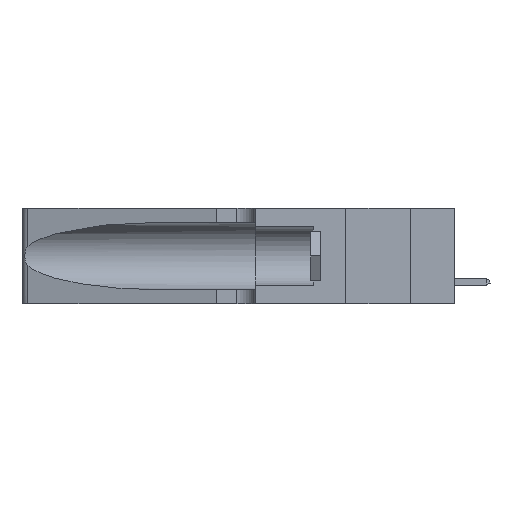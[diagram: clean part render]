
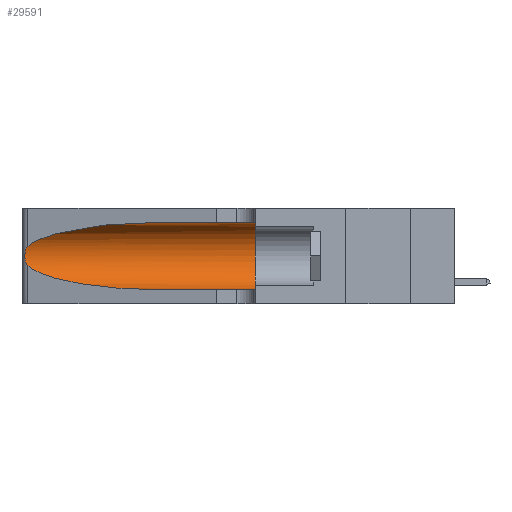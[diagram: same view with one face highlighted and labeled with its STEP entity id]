
A CAD part, left-side view. The second image highlights one B-rep face of the part: STEP entity #29591.
In plain terms, the highlighted cylindrical face has radius 3.308 mm (diameter 6.617 mm), a partial arc.
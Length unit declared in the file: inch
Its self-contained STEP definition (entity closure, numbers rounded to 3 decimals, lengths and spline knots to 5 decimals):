
#654 = CARTESIAN_POINT ( 'NONE',  ( 0.26018, 1.23835, 0.19895 ) ) ;
#2023 = CYLINDRICAL_SURFACE ( 'NONE', #17435, 0.13025 ) ;
#3804 = CARTESIAN_POINT ( 'NONE',  ( 0.25487, 1.22718, 0.14631 ) ) ;
#3829 = CARTESIAN_POINT ( 'NONE',  ( 0.25639, 1.23186, 0.15144 ) ) ;
#4115 = CARTESIAN_POINT ( 'NONE',  ( 0.25487, 1.22718, 0.14631 ) ) ;
#4376 = LINE ( 'NONE', #26707, #15599 ) ;
#4631 = CARTESIAN_POINT ( 'NONE',  ( 0.25487, 1.22718, 0.22369 ) ) ;
#6849 = CARTESIAN_POINT ( 'NONE',  ( 0.25789, 1.23486, 0.15765 ) ) ;
#6989 = CARTESIAN_POINT ( 'NONE',  ( 0.25787, 1.23484, 0.2124 ) ) ;
#7286 = DIRECTION ( 'NONE',  ( 0., -1., 0. ) ) ;
#7910 = CARTESIAN_POINT ( 'NONE',  ( 0.1305, 0.72297, 0.31525 ) ) ;
#8800 = DIRECTION ( 'NONE',  ( 0., 1., 0. ) ) ;
#9518 = VERTEX_POINT ( 'NONE', #11455 ) ;
#10012 = CARTESIAN_POINT ( 'NONE',  ( 0.26075, 1.23896, 0.178 ) ) ;
#10367 = DIRECTION ( 'NONE',  ( 0., -1., 0. ) ) ;
#11365 = ORIENTED_EDGE ( 'NONE', *, *, #36548, .T. ) ;
#11455 = CARTESIAN_POINT ( 'NONE',  ( 0.1305, 0.35, 0.05475 ) ) ;
#12756 = VECTOR ( 'NONE', #7286, 39.37008 ) ;
#12904 = CARTESIAN_POINT ( 'NONE',  ( 0.25555, 1.22994, 0.2215 ) ) ;
#13045 = CARTESIAN_POINT ( 'NONE',  ( 0.25555, 1.22993, 0.14849 ) ) ;
#13121 = ORIENTED_EDGE ( 'NONE', *, *, #21197, .T. ) ;
#13559 = CARTESIAN_POINT ( 'NONE',  ( 0.18966, 0.96281, 0.31525 ) ) ;
#14006 = CARTESIAN_POINT ( 'NONE',  ( 0.25487, 1.22718, 0.14631 ) ) ;
#14833 = CARTESIAN_POINT ( 'NONE',  ( 0.1305, 0.35, 0.31525 ) ) ;
#15152 = ORIENTED_EDGE ( 'NONE', *, *, #24577, .T. ) ;
#15599 = VECTOR ( 'NONE', #10367, 39.37008 ) ;
#15900 = CARTESIAN_POINT ( 'NONE',  ( 0.2373, 1.15595, 0.08982 ) ) ;
#15941 = CARTESIAN_POINT ( 'NONE',  ( 0.1305, 1.61858, 0.185 ) ) ;
#16346 = CARTESIAN_POINT ( 'NONE',  ( 0.1305, 1.61858, 0.31525 ) ) ;
#17435 = AXIS2_PLACEMENT_3D ( 'NONE', #15941, #22255, #37187 ) ;
#17780 = ORIENTED_EDGE ( 'NONE', *, *, #35893, .F. ) ;
#19254 = CARTESIAN_POINT ( 'NONE',  ( 0.26017, 1.23833, 0.17102 ) ) ;
#20992 = VERTEX_POINT ( 'NONE', #14006 ) ;
#21197 = EDGE_CURVE ( 'NONE', #20992, #29069, #37698, .T. ) ;
#21671 = CARTESIAN_POINT ( 'NONE',  ( 0.1305, 0.72297, 0.05475 ) ) ;
#22255 = DIRECTION ( 'NONE',  ( 0., -1., 0. ) ) ;
#22284 = AXIS2_PLACEMENT_3D ( 'NONE', #36166, #8800, #36276 ) ;
#24086 = FACE_OUTER_BOUND ( 'NONE', #31318, .T. ) ;
#24577 = EDGE_CURVE ( 'NONE', #36258, #20992, #36407, .T. ) ;
#25102 = CARTESIAN_POINT ( 'NONE',  ( 0.25856, 1.23593, 0.16098 ) ) ;
#26707 = CARTESIAN_POINT ( 'NONE',  ( 0.1305, 1.61858, 0.05475 ) ) ;
#27206 = ORIENTED_EDGE ( 'NONE', *, *, #30325, .F. ) ;
#27594 = VERTEX_POINT ( 'NONE', #38545 ) ;
#27685 = CARTESIAN_POINT ( 'NONE',  ( 0.25639, 1.23184, 0.21858 ) ) ;
#27833 = CARTESIAN_POINT ( 'NONE',  ( 0.25487, 1.22718, 0.22369 ) ) ;
#28887 = CARTESIAN_POINT ( 'NONE',  ( 0.2373, 1.15595, 0.28018 ) ) ;
#29069 = VERTEX_POINT ( 'NONE', #33826 ) ;
#29591 = ADVANCED_FACE ( 'NONE', ( #24086 ), #2023, .F. ) ;
#30109 = LINE ( 'NONE', #16346, #12756 ) ;
#30220 = CARTESIAN_POINT ( 'NONE',  ( 0.25487, 1.22718, 0.22369 ) ) ;
#30325 = EDGE_CURVE ( 'NONE', #27594, #36195, #30109, .T. ) ;
#31318 = EDGE_LOOP ( 'NONE', ( #36318, #15152, #13121, #11365, #17780, #27206 ) ) ;
#32387 =( BOUNDED_CURVE ( )  B_SPLINE_CURVE ( 3, ( #7910, #13559, #28887, #4631 ),
 .UNSPECIFIED., .F., .F. ) 
 B_SPLINE_CURVE_WITH_KNOTS ( ( 4, 4 ),
 ( 1.5708, 2.84003 ),
 .UNSPECIFIED. ) 
 CURVE ( )  GEOMETRIC_REPRESENTATION_ITEM ( )  RATIONAL_B_SPLINE_CURVE ( ( 1., 0.87, 0.87, 1. ) ) 
 REPRESENTATION_ITEM ( '' )  );
#32935 = EDGE_CURVE ( 'NONE', #27594, #36258, #32387, .T. ) ;
#33427 = CARTESIAN_POINT ( 'NONE',  ( 0.18966, 0.96281, 0.05475 ) ) ;
#33826 = CARTESIAN_POINT ( 'NONE',  ( 0.1305, 0.72297, 0.05475 ) ) ;
#33984 = CIRCLE ( 'NONE', #22284, 0.13025 ) ;
#35893 = EDGE_CURVE ( 'NONE', #36195, #9518, #33984, .T. ) ;
#36166 = CARTESIAN_POINT ( 'NONE',  ( 0.1305, 0.35, 0.185 ) ) ;
#36195 = VERTEX_POINT ( 'NONE', #14833 ) ;
#36258 = VERTEX_POINT ( 'NONE', #30220 ) ;
#36276 = DIRECTION ( 'NONE',  ( 0., 0., 1. ) ) ;
#36318 = ORIENTED_EDGE ( 'NONE', *, *, #32935, .T. ) ;
#36407 = B_SPLINE_CURVE_WITH_KNOTS ( 'NONE', 3,
 ( #27833, #12904, #27685, #6989, #37173, #654, #37036, #10012, #19254, #25102, #6849, #3829, #13045, #4115 ),
 .UNSPECIFIED., .F., .F.,
 ( 4, 2, 2, 2, 2, 2, 4 ),
 ( 0., 0.00027, 0.00053, 0.00107, 0.0016, 0.00187, 0.00214 ),
 .UNSPECIFIED. ) ;
#36548 = EDGE_CURVE ( 'NONE', #29069, #9518, #4376, .T. ) ;
#37036 = CARTESIAN_POINT ( 'NONE',  ( 0.26075, 1.23896, 0.19203 ) ) ;
#37173 = CARTESIAN_POINT ( 'NONE',  ( 0.25854, 1.2359, 0.20912 ) ) ;
#37187 = DIRECTION ( 'NONE',  ( 0., 0., -1. ) ) ;
#37698 =( BOUNDED_CURVE ( )  B_SPLINE_CURVE ( 3, ( #3804, #15900, #33427, #21671 ),
 .UNSPECIFIED., .F., .F. ) 
 B_SPLINE_CURVE_WITH_KNOTS ( ( 4, 4 ),
 ( 3.44316, 4.71239 ),
 .UNSPECIFIED. ) 
 CURVE ( )  GEOMETRIC_REPRESENTATION_ITEM ( )  RATIONAL_B_SPLINE_CURVE ( ( 1., 0.87, 0.87, 1. ) ) 
 REPRESENTATION_ITEM ( '' )  );
#38545 = CARTESIAN_POINT ( 'NONE',  ( 0.1305, 0.72297, 0.31525 ) ) ;
